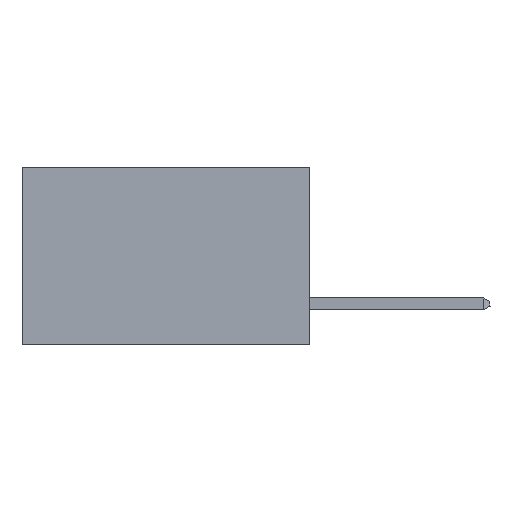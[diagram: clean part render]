
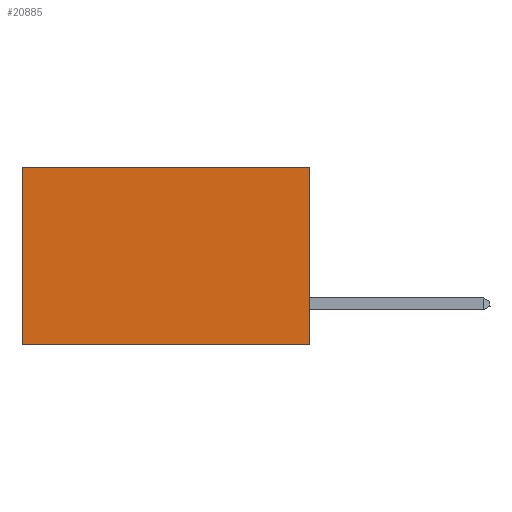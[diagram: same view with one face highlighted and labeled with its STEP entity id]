
A CAD part, left-side view. The second image highlights one B-rep face of the part: STEP entity #20885.
In plain terms, the highlighted planar face has unit normal (-1, 0, 0).
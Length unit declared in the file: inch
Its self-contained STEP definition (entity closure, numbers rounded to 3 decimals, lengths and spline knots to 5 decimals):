
#110 = DIRECTION ( 'NONE',  ( 1., 0., 0. ) ) ;
#1786 = EDGE_CURVE ( 'NONE', #23947, #23055, #11137, .T. ) ;
#2403 = LINE ( 'NONE', #7340, #3457 ) ;
#2490 = ORIENTED_EDGE ( 'NONE', *, *, #1786, .F. ) ;
#3457 = VECTOR ( 'NONE', #24054, 39.37008 ) ;
#4069 = ORIENTED_EDGE ( 'NONE', *, *, #24346, .F. ) ;
#4443 = VERTEX_POINT ( 'NONE', #5164 ) ;
#4637 = DIRECTION ( 'NONE',  ( 0., 1., 0. ) ) ;
#4803 = VERTEX_POINT ( 'NONE', #22380 ) ;
#5164 = CARTESIAN_POINT ( 'NONE',  ( 0.2875, 0.6, -0.37 ) ) ;
#7340 = CARTESIAN_POINT ( 'NONE',  ( 0.2875, 0.6, 0. ) ) ;
#9177 = CARTESIAN_POINT ( 'NONE',  ( 0.2875, 0., -0.37 ) ) ;
#11031 = CARTESIAN_POINT ( 'NONE',  ( 0.2875, 0., 0. ) ) ;
#11137 = LINE ( 'NONE', #16689, #26824 ) ;
#12620 = PLANE ( 'NONE',  #15858 ) ;
#13058 = LINE ( 'NONE', #24328, #22404 ) ;
#13153 = DIRECTION ( 'NONE',  ( 0., 0., -1. ) ) ;
#13404 = ORIENTED_EDGE ( 'NONE', *, *, #21539, .T. ) ;
#15369 = CARTESIAN_POINT ( 'NONE',  ( 0.2875, 0., 0. ) ) ;
#15858 = AXIS2_PLACEMENT_3D ( 'NONE', #11031, #110, #13153 ) ;
#16689 = CARTESIAN_POINT ( 'NONE',  ( 0.2875, 0., 0. ) ) ;
#16962 = DIRECTION ( 'NONE',  ( 0., 0., -1. ) ) ;
#16965 = EDGE_CURVE ( 'NONE', #4803, #4443, #2403, .T. ) ;
#18830 = FACE_OUTER_BOUND ( 'NONE', #26201, .T. ) ;
#20404 = DIRECTION ( 'NONE',  ( 0., 1., 0. ) ) ;
#20787 = VECTOR ( 'NONE', #4637, 39.37008 ) ;
#20885 = ADVANCED_FACE ( 'NONE', ( #18830 ), #12620, .F. ) ;
#21125 = LINE ( 'NONE', #15369, #20787 ) ;
#21539 = EDGE_CURVE ( 'NONE', #23947, #4803, #21125, .T. ) ;
#22380 = CARTESIAN_POINT ( 'NONE',  ( 0.2875, 0.6, 0. ) ) ;
#22404 = VECTOR ( 'NONE', #20404, 39.37008 ) ;
#22720 = ORIENTED_EDGE ( 'NONE', *, *, #16965, .T. ) ;
#23055 = VERTEX_POINT ( 'NONE', #9177 ) ;
#23947 = VERTEX_POINT ( 'NONE', #25378 ) ;
#24054 = DIRECTION ( 'NONE',  ( 0., 0., -1. ) ) ;
#24328 = CARTESIAN_POINT ( 'NONE',  ( 0.2875, 0., -0.37 ) ) ;
#24346 = EDGE_CURVE ( 'NONE', #23055, #4443, #13058, .T. ) ;
#25378 = CARTESIAN_POINT ( 'NONE',  ( 0.2875, 0., 0. ) ) ;
#26201 = EDGE_LOOP ( 'NONE', ( #22720, #4069, #2490, #13404 ) ) ;
#26824 = VECTOR ( 'NONE', #16962, 39.37008 ) ;
